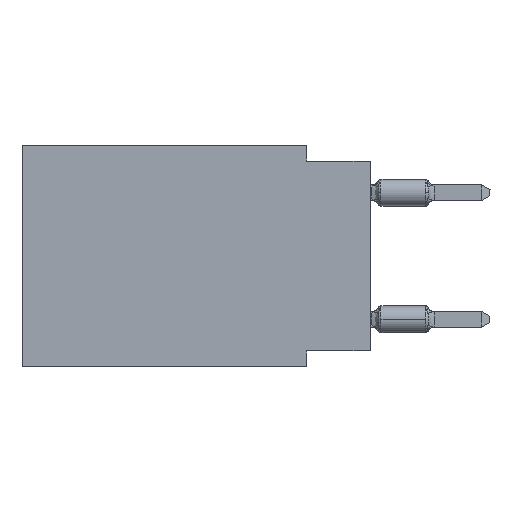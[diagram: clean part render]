
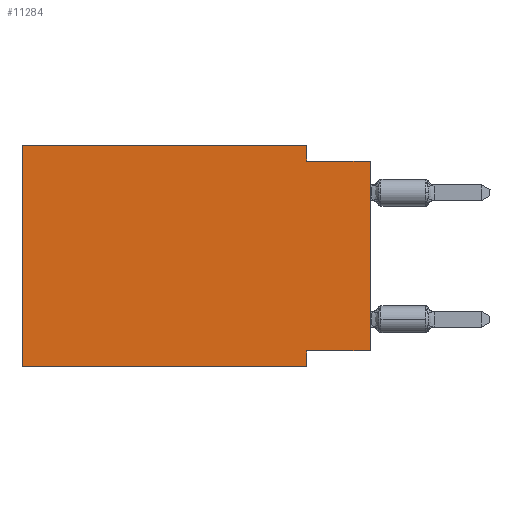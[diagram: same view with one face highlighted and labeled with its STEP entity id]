
A CAD part, left-side view. The second image highlights one B-rep face of the part: STEP entity #11284.
In plain terms, the highlighted planar face has unit normal (-1, 0, 0).
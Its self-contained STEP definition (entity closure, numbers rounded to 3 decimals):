
#321 = VECTOR ( 'NONE', #28742, 1000. ) ;
#423 = DIRECTION ( 'NONE',  ( 0., 0., -1. ) ) ;
#777 = ORIENTED_EDGE ( 'NONE', *, *, #29223, .T. ) ;
#1676 = VERTEX_POINT ( 'NONE', #29974 ) ;
#2280 = EDGE_CURVE ( 'NONE', #31260, #41338, #3633, .T. ) ;
#2497 = ORIENTED_EDGE ( 'NONE', *, *, #3134, .F. ) ;
#3134 = EDGE_CURVE ( 'NONE', #4184, #14137, #38849, .T. ) ;
#3199 = PLANE ( 'NONE',  #24163 ) ;
#3211 = VECTOR ( 'NONE', #6743, 1000. ) ;
#3633 = LINE ( 'NONE', #25977, #10670 ) ;
#3747 = CARTESIAN_POINT ( 'NONE',  ( 0., 13.97, 0. ) ) ;
#3913 = VECTOR ( 'NONE', #26582, 1000. ) ;
#4037 = LINE ( 'NONE', #36775, #3913 ) ;
#4053 = DIRECTION ( 'NONE',  ( 0., 0., -1. ) ) ;
#4157 = VERTEX_POINT ( 'NONE', #22284 ) ;
#4184 = VERTEX_POINT ( 'NONE', #25449 ) ;
#5144 = CARTESIAN_POINT ( 'NONE',  ( 0., 0., -0.635 ) ) ;
#5643 = DIRECTION ( 'NONE',  ( 0., -1., 0. ) ) ;
#6278 = CARTESIAN_POINT ( 'NONE',  ( 0., 13.97, 0. ) ) ;
#6638 = DIRECTION ( 'NONE',  ( 0., 1., 0. ) ) ;
#6743 = DIRECTION ( 'NONE',  ( 0., 0., 1. ) ) ;
#6989 = VECTOR ( 'NONE', #8678, 1000. ) ;
#8678 = DIRECTION ( 'NONE',  ( 0., 0., -1. ) ) ;
#8964 = CARTESIAN_POINT ( 'NONE',  ( 0., 13.97, 0. ) ) ;
#9403 = CARTESIAN_POINT ( 'NONE',  ( 0., 13.97, 0. ) ) ;
#10437 = CARTESIAN_POINT ( 'NONE',  ( 0., 2.54, 0. ) ) ;
#10670 = VECTOR ( 'NONE', #6638, 1000. ) ;
#10682 = ORIENTED_EDGE ( 'NONE', *, *, #2280, .F. ) ;
#11284 = ADVANCED_FACE ( 'NONE', ( #19360 ), #3199, .F. ) ;
#12082 = CARTESIAN_POINT ( 'NONE',  ( 0., 2.54, -8.89 ) ) ;
#12853 = ORIENTED_EDGE ( 'NONE', *, *, #25967, .F. ) ;
#13133 = VECTOR ( 'NONE', #4053, 1000. ) ;
#13900 = ORIENTED_EDGE ( 'NONE', *, *, #32528, .F. ) ;
#14137 = VERTEX_POINT ( 'NONE', #6278 ) ;
#14450 = EDGE_CURVE ( 'NONE', #31260, #19610, #4037, .T. ) ;
#15248 = LINE ( 'NONE', #12082, #6989 ) ;
#15814 = EDGE_LOOP ( 'NONE', ( #17821, #13900, #19328, #12853, #2497, #777, #38591, #10682 ) ) ;
#17286 = CARTESIAN_POINT ( 'NONE',  ( 0., 0., -8.255 ) ) ;
#17821 = ORIENTED_EDGE ( 'NONE', *, *, #14450, .T. ) ;
#19328 = ORIENTED_EDGE ( 'NONE', *, *, #36715, .F. ) ;
#19360 = FACE_OUTER_BOUND ( 'NONE', #15814, .T. ) ;
#19610 = VERTEX_POINT ( 'NONE', #5144 ) ;
#21192 = LINE ( 'NONE', #31383, #36199 ) ;
#22284 = CARTESIAN_POINT ( 'NONE',  ( 0., 2.54, -8.89 ) ) ;
#22634 = CARTESIAN_POINT ( 'NONE',  ( 0., 2.54, -0.635 ) ) ;
#24163 = AXIS2_PLACEMENT_3D ( 'NONE', #8964, #34902, #423 ) ;
#25449 = CARTESIAN_POINT ( 'NONE',  ( 0., 13.97, -8.89 ) ) ;
#25967 = EDGE_CURVE ( 'NONE', #14137, #1676, #29159, .T. ) ;
#25977 = CARTESIAN_POINT ( 'NONE',  ( 0., 0., -8.255 ) ) ;
#26582 = DIRECTION ( 'NONE',  ( 0., 0., 1. ) ) ;
#27573 = VECTOR ( 'NONE', #39875, 1000. ) ;
#28742 = DIRECTION ( 'NONE',  ( 0., -1., 0. ) ) ;
#29159 = LINE ( 'NONE', #9403, #321 ) ;
#29223 = EDGE_CURVE ( 'NONE', #4184, #4157, #36689, .T. ) ;
#29974 = CARTESIAN_POINT ( 'NONE',  ( 0., 2.54, 0. ) ) ;
#31260 = VERTEX_POINT ( 'NONE', #17286 ) ;
#31383 = CARTESIAN_POINT ( 'NONE',  ( 0., 0., -0.635 ) ) ;
#31486 = VERTEX_POINT ( 'NONE', #22634 ) ;
#32528 = EDGE_CURVE ( 'NONE', #31486, #19610, #21192, .T. ) ;
#34549 = CARTESIAN_POINT ( 'NONE',  ( 0., 2.54, -8.255 ) ) ;
#34902 = DIRECTION ( 'NONE',  ( 1., 0., 0. ) ) ;
#36199 = VECTOR ( 'NONE', #5643, 1000. ) ;
#36260 = CARTESIAN_POINT ( 'NONE',  ( 0., 13.97, -8.89 ) ) ;
#36360 = LINE ( 'NONE', #10437, #13133 ) ;
#36689 = LINE ( 'NONE', #36260, #27573 ) ;
#36715 = EDGE_CURVE ( 'NONE', #1676, #31486, #36360, .T. ) ;
#36775 = CARTESIAN_POINT ( 'NONE',  ( 0., 0., 0. ) ) ;
#37960 = EDGE_CURVE ( 'NONE', #41338, #4157, #15248, .T. ) ;
#38591 = ORIENTED_EDGE ( 'NONE', *, *, #37960, .F. ) ;
#38849 = LINE ( 'NONE', #3747, #3211 ) ;
#39875 = DIRECTION ( 'NONE',  ( 0., -1., 0. ) ) ;
#41338 = VERTEX_POINT ( 'NONE', #34549 ) ;
